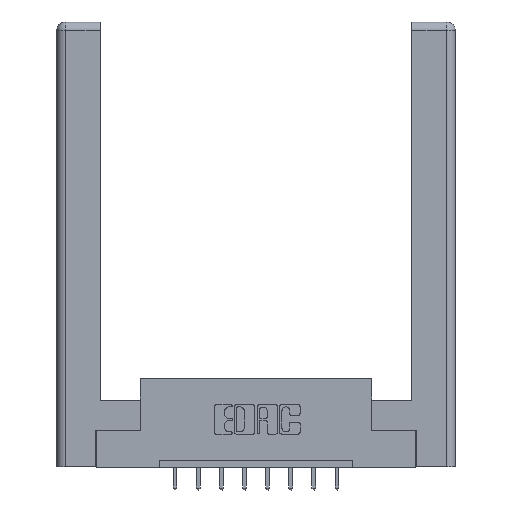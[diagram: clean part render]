
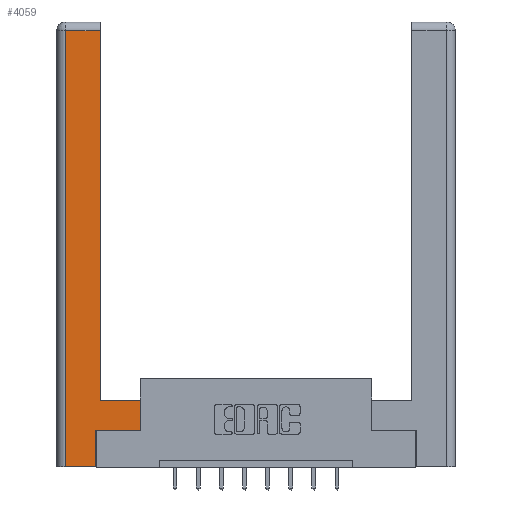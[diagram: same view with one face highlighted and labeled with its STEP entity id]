
A CAD part, top view. The second image highlights one B-rep face of the part: STEP entity #4059.
In plain terms, the highlighted planar face has unit normal (0, 0, 1).
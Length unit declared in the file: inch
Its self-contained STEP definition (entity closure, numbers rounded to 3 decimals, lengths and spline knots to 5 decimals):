
#14 = CARTESIAN_POINT ( 'NONE',  ( 0.565, 0.245, 0. ) ) ;
#75 = ORIENTED_EDGE ( 'NONE', *, *, #9926, .T. ) ;
#80 = ORIENTED_EDGE ( 'NONE', *, *, #4742, .T. ) ;
#136 = CARTESIAN_POINT ( 'NONE',  ( 0., 0., 0. ) ) ;
#471 = ORIENTED_EDGE ( 'NONE', *, *, #4531, .T. ) ;
#519 = VECTOR ( 'NONE', #3037, 39.37008 ) ;
#1100 = LINE ( 'NONE', #4608, #6399 ) ;
#1124 = DIRECTION ( 'NONE',  ( 1., 0., 0. ) ) ;
#1350 = VECTOR ( 'NONE', #6740, 39.37008 ) ;
#2050 = CARTESIAN_POINT ( 'NONE',  ( 0.0615, 2.94, 0. ) ) ;
#2632 = ORIENTED_EDGE ( 'NONE', *, *, #11240, .T. ) ;
#3037 = DIRECTION ( 'NONE',  ( 0., 1., 0. ) ) ;
#3180 = EDGE_CURVE ( 'NONE', #5938, #9607, #5562, .T. ) ;
#3196 = DIRECTION ( 'NONE',  ( -1., 0., 0. ) ) ;
#3491 = ORIENTED_EDGE ( 'NONE', *, *, #3180, .T. ) ;
#3806 = DIRECTION ( 'NONE',  ( 0., 1., 0. ) ) ;
#3977 = ORIENTED_EDGE ( 'NONE', *, *, #11438, .T. ) ;
#4059 = ADVANCED_FACE ( 'NONE', ( #10402 ), #8122, .F. ) ;
#4255 = VERTEX_POINT ( 'NONE', #4755 ) ;
#4360 = CARTESIAN_POINT ( 'NONE',  ( 0.295, 3., 0. ) ) ;
#4396 = CARTESIAN_POINT ( 'NONE',  ( 0.265, 0.245, 0. ) ) ;
#4429 = EDGE_LOOP ( 'NONE', ( #5700, #471, #10090, #75, #2632, #3977, #80, #3491 ) ) ;
#4458 = LINE ( 'NONE', #6921, #9358 ) ;
#4488 = DIRECTION ( 'NONE',  ( 1., 0., 0. ) ) ;
#4531 = EDGE_CURVE ( 'NONE', #5992, #9790, #1100, .T. ) ;
#4608 = CARTESIAN_POINT ( 'NONE',  ( 0.0615, 2.94, 0. ) ) ;
#4674 = LINE ( 'NONE', #12650, #11482 ) ;
#4742 = EDGE_CURVE ( 'NONE', #9062, #5938, #4851, .T. ) ;
#4755 = CARTESIAN_POINT ( 'NONE',  ( 0.265, 0.245, 0. ) ) ;
#4781 = CARTESIAN_POINT ( 'NONE',  ( 0.265, 0., 0. ) ) ;
#4851 = LINE ( 'NONE', #12828, #5156 ) ;
#5156 = VECTOR ( 'NONE', #11213, 39.37008 ) ;
#5158 = EDGE_CURVE ( 'NONE', #9790, #10075, #4674, .T. ) ;
#5562 = LINE ( 'NONE', #11734, #1350 ) ;
#5700 = ORIENTED_EDGE ( 'NONE', *, *, #6882, .T. ) ;
#5938 = VERTEX_POINT ( 'NONE', #9888 ) ;
#5992 = VERTEX_POINT ( 'NONE', #8908 ) ;
#6399 = VECTOR ( 'NONE', #10752, 39.37008 ) ;
#6426 = LINE ( 'NONE', #4360, #519 ) ;
#6628 = CARTESIAN_POINT ( 'NONE',  ( 0.265, 0., 0. ) ) ;
#6740 = DIRECTION ( 'NONE',  ( -1., 0., 0. ) ) ;
#6882 = EDGE_CURVE ( 'NONE', #9607, #5992, #6426, .T. ) ;
#6921 = CARTESIAN_POINT ( 'NONE',  ( 0.565, 0.245, 0. ) ) ;
#8122 = PLANE ( 'NONE',  #8489 ) ;
#8489 = AXIS2_PLACEMENT_3D ( 'NONE', #136, #11209, #3196 ) ;
#8908 = CARTESIAN_POINT ( 'NONE',  ( 0.295, 2.94, 0. ) ) ;
#9062 = VERTEX_POINT ( 'NONE', #14 ) ;
#9358 = VECTOR ( 'NONE', #1124, 39.37008 ) ;
#9607 = VERTEX_POINT ( 'NONE', #10986 ) ;
#9702 = LINE ( 'NONE', #6628, #12537 ) ;
#9790 = VERTEX_POINT ( 'NONE', #2050 ) ;
#9888 = CARTESIAN_POINT ( 'NONE',  ( 0.565, 0.45, 0. ) ) ;
#9926 = EDGE_CURVE ( 'NONE', #10075, #12754, #9702, .T. ) ;
#10075 = VERTEX_POINT ( 'NONE', #11777 ) ;
#10090 = ORIENTED_EDGE ( 'NONE', *, *, #5158, .T. ) ;
#10402 = FACE_OUTER_BOUND ( 'NONE', #4429, .T. ) ;
#10615 = DIRECTION ( 'NONE',  ( 0., -1., 0. ) ) ;
#10752 = DIRECTION ( 'NONE',  ( -1., 0., 0. ) ) ;
#10973 = VECTOR ( 'NONE', #3806, 39.37008 ) ;
#10986 = CARTESIAN_POINT ( 'NONE',  ( 0.295, 0.45, 0. ) ) ;
#11209 = DIRECTION ( 'NONE',  ( 0., 0., -1. ) ) ;
#11213 = DIRECTION ( 'NONE',  ( 0., 1., 0. ) ) ;
#11240 = EDGE_CURVE ( 'NONE', #12754, #4255, #12200, .T. ) ;
#11438 = EDGE_CURVE ( 'NONE', #4255, #9062, #4458, .T. ) ;
#11482 = VECTOR ( 'NONE', #10615, 39.37008 ) ;
#11734 = CARTESIAN_POINT ( 'NONE',  ( 0.295, 0.45, 0. ) ) ;
#11777 = CARTESIAN_POINT ( 'NONE',  ( 0.0615, 0., 0. ) ) ;
#12200 = LINE ( 'NONE', #4396, #10973 ) ;
#12537 = VECTOR ( 'NONE', #4488, 39.37008 ) ;
#12650 = CARTESIAN_POINT ( 'NONE',  ( 0.0615, 0., 0. ) ) ;
#12754 = VERTEX_POINT ( 'NONE', #4781 ) ;
#12828 = CARTESIAN_POINT ( 'NONE',  ( 0.565, 0.45, 0. ) ) ;
